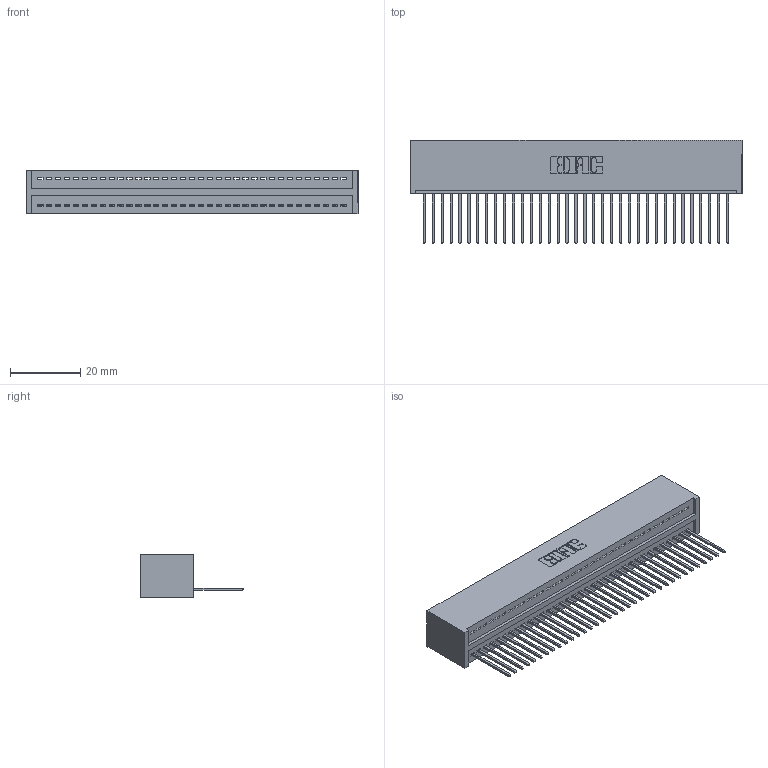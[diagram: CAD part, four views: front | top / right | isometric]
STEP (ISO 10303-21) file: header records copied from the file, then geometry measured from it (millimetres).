
FILE_DESCRIPTION (( 'STEP AP203' ), '1' );
FILE_NAME ('325-035-540-101.STEP', '2020-02-24T20:17:52', ( '' ), ( '' ), 'SwSTEP 2.0', 'SolidWorks 2016', '' );
FILE_SCHEMA (( 'CONFIG_CONTROL_DESIGN' ));
Length unit declared in the file: inch
Products named in the file (3): 325 Part_Lugless; 325-035-540-101; 325-292-001_325-293-140
Assembly tree (36 placements, depth 2):
  325-035-540-101
    325 Part_Lugless
    325-292-001_325-293-140  x35
Bounding box: 94.54 x 29.46 x 12.45 mm (x, y, z)
Volume: 12565.9 mm3; surface area: 14450.4 mm2
Topology: 36 solids, 36 shells, 2136 faces, 6447 edges, 4250 vertices
Faces by surface type: plane 1536, cylinder 600
Entity records: 22043 total; most frequent: CARTESIAN_POINT 3811, ORIENTED_EDGE 3782, DIRECTION 3221, EDGE_CURVE 1891, VECTOR 1771, LINE 1771, VERTEX_POINT 1258, AXIS2_PLACEMENT_3D 725
